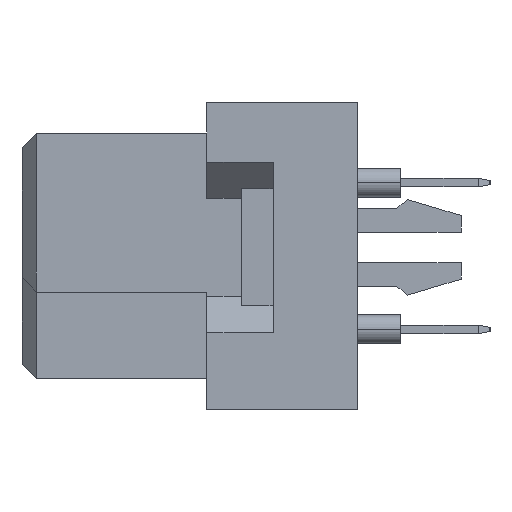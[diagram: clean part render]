
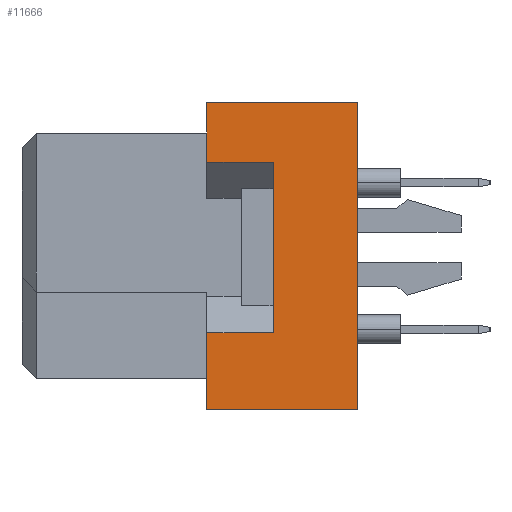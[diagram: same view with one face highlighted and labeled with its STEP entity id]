
A CAD part, left-side view. The second image highlights one B-rep face of the part: STEP entity #11666.
In plain terms, the highlighted planar face has unit normal (-1, 0, 0).
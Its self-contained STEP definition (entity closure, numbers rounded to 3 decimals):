
#363 = CARTESIAN_POINT ( 'NONE',  ( -27.5, -6.4, 5.3 ) ) ;
#686 = CARTESIAN_POINT ( 'NONE',  ( -27.5, -11.6, -5.3 ) ) ;
#788 = ORIENTED_EDGE ( 'NONE', *, *, #12408, .T. ) ;
#1036 = VERTEX_POINT ( 'NONE', #7702 ) ;
#1139 = LINE ( 'NONE', #10248, #10440 ) ;
#1296 = VECTOR ( 'NONE', #12720, 1000. ) ;
#1414 = VECTOR ( 'NONE', #11973, 1000. ) ;
#1608 = EDGE_CURVE ( 'NONE', #2904, #14873, #8120, .T. ) ;
#1620 = VECTOR ( 'NONE', #14720, 1000. ) ;
#1742 = LINE ( 'NONE', #20407, #1414 ) ;
#2286 = VERTEX_POINT ( 'NONE', #686 ) ;
#2528 = VERTEX_POINT ( 'NONE', #8501 ) ;
#2904 = VERTEX_POINT ( 'NONE', #15361 ) ;
#3112 = VECTOR ( 'NONE', #11751, 1000. ) ;
#3258 = ORIENTED_EDGE ( 'NONE', *, *, #13646, .F. ) ;
#3494 = CARTESIAN_POINT ( 'NONE',  ( -27.5, -11.6, -5.3 ) ) ;
#3570 = PLANE ( 'NONE',  #16148 ) ;
#4523 = CARTESIAN_POINT ( 'NONE',  ( -27.5, -8.7, 3.25 ) ) ;
#4788 = CARTESIAN_POINT ( 'NONE',  ( -27.5, -6.4, -5.3 ) ) ;
#5031 = CARTESIAN_POINT ( 'NONE',  ( -27.5, -8.7, 3.25 ) ) ;
#5758 = VERTEX_POINT ( 'NONE', #363 ) ;
#6157 = DIRECTION ( 'NONE',  ( -1., 0., 0. ) ) ;
#6889 = VECTOR ( 'NONE', #16191, 1000. ) ;
#6915 = CARTESIAN_POINT ( 'NONE',  ( -27.5, -6.4, -2.65 ) ) ;
#7702 = CARTESIAN_POINT ( 'NONE',  ( -27.5, -6.4, 3.25 ) ) ;
#7911 = ORIENTED_EDGE ( 'NONE', *, *, #19802, .F. ) ;
#7974 = DIRECTION ( 'NONE',  ( 0., 1., 0. ) ) ;
#8029 = EDGE_LOOP ( 'NONE', ( #788, #13761, #3258, #20577, #8688, #7911, #16152, #14230 ) ) ;
#8120 = LINE ( 'NONE', #4788, #1620 ) ;
#8143 = LINE ( 'NONE', #21502, #17494 ) ;
#8501 = CARTESIAN_POINT ( 'NONE',  ( -27.5, -8.7, -2.65 ) ) ;
#8688 = ORIENTED_EDGE ( 'NONE', *, *, #14235, .T. ) ;
#9493 = LINE ( 'NONE', #12910, #6889 ) ;
#10119 = EDGE_CURVE ( 'NONE', #18091, #1036, #20086, .T. ) ;
#10151 = EDGE_CURVE ( 'NONE', #2528, #18091, #8143, .T. ) ;
#10218 = DIRECTION ( 'NONE',  ( 0., 1., 0. ) ) ;
#10248 = CARTESIAN_POINT ( 'NONE',  ( -27.5, -11.6, 5.3 ) ) ;
#10440 = VECTOR ( 'NONE', #7974, 1000. ) ;
#10801 = DIRECTION ( 'NONE',  ( 0., 0., 1. ) ) ;
#11666 = ADVANCED_FACE ( 'NONE', ( #18636 ), #3570, .T. ) ;
#11751 = DIRECTION ( 'NONE',  ( 0., 1., 0. ) ) ;
#11862 = LINE ( 'NONE', #3494, #14280 ) ;
#11973 = DIRECTION ( 'NONE',  ( 0., 1., 0. ) ) ;
#12304 = DIRECTION ( 'NONE',  ( 0., 0., 1. ) ) ;
#12408 = EDGE_CURVE ( 'NONE', #2528, #14873, #1742, .T. ) ;
#12720 = DIRECTION ( 'NONE',  ( 0., 0., 1. ) ) ;
#12823 = CARTESIAN_POINT ( 'NONE',  ( -27.5, -11.6, 5.3 ) ) ;
#12910 = CARTESIAN_POINT ( 'NONE',  ( -27.5, -6.4, -5.3 ) ) ;
#13049 = LINE ( 'NONE', #12823, #1296 ) ;
#13646 = EDGE_CURVE ( 'NONE', #2286, #2904, #11862, .T. ) ;
#13761 = ORIENTED_EDGE ( 'NONE', *, *, #1608, .F. ) ;
#14230 = ORIENTED_EDGE ( 'NONE', *, *, #10151, .F. ) ;
#14235 = EDGE_CURVE ( 'NONE', #17752, #5758, #1139, .T. ) ;
#14280 = VECTOR ( 'NONE', #10218, 1000. ) ;
#14720 = DIRECTION ( 'NONE',  ( 0., 0., 1. ) ) ;
#14873 = VERTEX_POINT ( 'NONE', #6915 ) ;
#15361 = CARTESIAN_POINT ( 'NONE',  ( -27.5, -6.4, -5.3 ) ) ;
#16148 = AXIS2_PLACEMENT_3D ( 'NONE', #20990, #6157, #10801 ) ;
#16152 = ORIENTED_EDGE ( 'NONE', *, *, #10119, .F. ) ;
#16191 = DIRECTION ( 'NONE',  ( 0., 0., 1. ) ) ;
#16308 = CARTESIAN_POINT ( 'NONE',  ( -27.5, -11.6, 5.3 ) ) ;
#17494 = VECTOR ( 'NONE', #12304, 1000. ) ;
#17752 = VERTEX_POINT ( 'NONE', #16308 ) ;
#18091 = VERTEX_POINT ( 'NONE', #4523 ) ;
#18636 = FACE_OUTER_BOUND ( 'NONE', #8029, .T. ) ;
#19802 = EDGE_CURVE ( 'NONE', #1036, #5758, #9493, .T. ) ;
#20086 = LINE ( 'NONE', #5031, #3112 ) ;
#20407 = CARTESIAN_POINT ( 'NONE',  ( -27.5, -8.7, -2.65 ) ) ;
#20577 = ORIENTED_EDGE ( 'NONE', *, *, #20692, .T. ) ;
#20692 = EDGE_CURVE ( 'NONE', #2286, #17752, #13049, .T. ) ;
#20990 = CARTESIAN_POINT ( 'NONE',  ( -27.5, -11.6, 5.3 ) ) ;
#21502 = CARTESIAN_POINT ( 'NONE',  ( -27.5, -8.7, -2.65 ) ) ;
